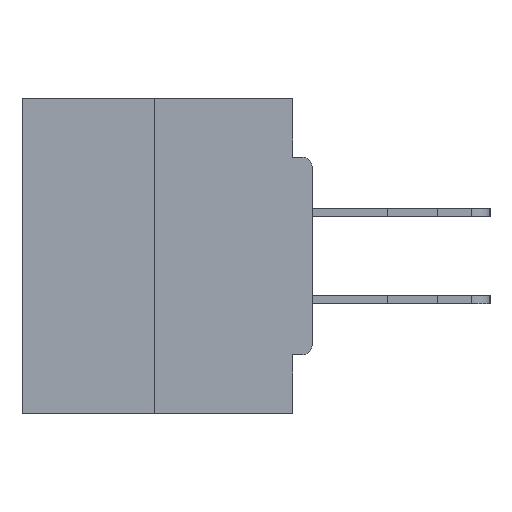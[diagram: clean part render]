
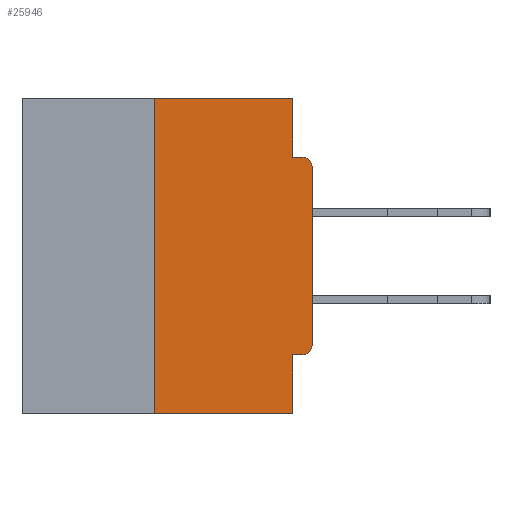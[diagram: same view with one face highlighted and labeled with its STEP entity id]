
A CAD part, left-side view. The second image highlights one B-rep face of the part: STEP entity #25946.
In plain terms, the highlighted planar face has unit normal (-1, 0, 0).
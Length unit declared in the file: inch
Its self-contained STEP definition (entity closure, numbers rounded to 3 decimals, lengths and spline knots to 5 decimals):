
#322 = VECTOR ( 'NONE', #29726, 39.37008 ) ;
#1037 = VERTEX_POINT ( 'NONE', #26358 ) ;
#1400 = VECTOR ( 'NONE', #1673, 39.37008 ) ;
#1673 = DIRECTION ( 'NONE',  ( 0., 0., -1. ) ) ;
#1866 = CARTESIAN_POINT ( 'NONE',  ( 0., 0.031, -0.5 ) ) ;
#2128 = CARTESIAN_POINT ( 'NONE',  ( 0., 0.25, -0.5 ) ) ;
#3166 = LINE ( 'NONE', #31218, #36652 ) ;
#3192 = VERTEX_POINT ( 'NONE', #12586 ) ;
#3571 = VECTOR ( 'NONE', #27977, 39.37008 ) ;
#4007 = VERTEX_POINT ( 'NONE', #32716 ) ;
#4703 = EDGE_LOOP ( 'NONE', ( #18840, #27995, #8814, #18042, #5369, #9398, #6115, #21637, #16506, #18083 ) ) ;
#5052 = VERTEX_POINT ( 'NONE', #2128 ) ;
#5257 = AXIS2_PLACEMENT_3D ( 'NONE', #32808, #23676, #10873 ) ;
#5369 = ORIENTED_EDGE ( 'NONE', *, *, #29770, .F. ) ;
#6115 = ORIENTED_EDGE ( 'NONE', *, *, #11020, .T. ) ;
#6342 = DIRECTION ( 'NONE',  ( 0., 1., 0. ) ) ;
#6436 = CARTESIAN_POINT ( 'NONE',  ( 0., 0.031, -0.0935 ) ) ;
#7241 = CIRCLE ( 'NONE', #5257, 0.015 ) ;
#7997 = VERTEX_POINT ( 'NONE', #20599 ) ;
#8484 = CIRCLE ( 'NONE', #36384, 0.015 ) ;
#8524 = DIRECTION ( 'NONE',  ( 0., 0., -1. ) ) ;
#8814 = ORIENTED_EDGE ( 'NONE', *, *, #34856, .T. ) ;
#8914 = PLANE ( 'NONE',  #25344 ) ;
#9200 = VERTEX_POINT ( 'NONE', #6436 ) ;
#9283 = EDGE_CURVE ( 'NONE', #3192, #9200, #27256, .T. ) ;
#9398 = ORIENTED_EDGE ( 'NONE', *, *, #17952, .T. ) ;
#9691 = DIRECTION ( 'NONE',  ( -1., 0., 0. ) ) ;
#10873 = DIRECTION ( 'NONE',  ( 0., 0., -1. ) ) ;
#11020 = EDGE_CURVE ( 'NONE', #1037, #33660, #17068, .T. ) ;
#12321 = CARTESIAN_POINT ( 'NONE',  ( 0., 0.46, -0.5 ) ) ;
#12525 = VERTEX_POINT ( 'NONE', #18165 ) ;
#12586 = CARTESIAN_POINT ( 'NONE',  ( 0., 0.031, 0. ) ) ;
#16506 = ORIENTED_EDGE ( 'NONE', *, *, #16971, .F. ) ;
#16971 = EDGE_CURVE ( 'NONE', #9200, #12525, #34579, .T. ) ;
#17068 = LINE ( 'NONE', #26404, #28791 ) ;
#17894 = CARTESIAN_POINT ( 'NONE',  ( 0., 0.46, 0. ) ) ;
#17921 = DIRECTION ( 'NONE',  ( 0., 0., -1. ) ) ;
#17952 = EDGE_CURVE ( 'NONE', #7997, #1037, #8484, .T. ) ;
#18042 = ORIENTED_EDGE ( 'NONE', *, *, #27162, .F. ) ;
#18083 = ORIENTED_EDGE ( 'NONE', *, *, #9283, .F. ) ;
#18100 = FACE_OUTER_BOUND ( 'NONE', #4703, .T. ) ;
#18165 = CARTESIAN_POINT ( 'NONE',  ( 0., 0.015, -0.0935 ) ) ;
#18563 = VERTEX_POINT ( 'NONE', #33606 ) ;
#18840 = ORIENTED_EDGE ( 'NONE', *, *, #23369, .F. ) ;
#19565 = DIRECTION ( 'NONE',  ( 0., -1., 0. ) ) ;
#19803 = CARTESIAN_POINT ( 'NONE',  ( 0., 0.25, 0. ) ) ;
#20599 = CARTESIAN_POINT ( 'NONE',  ( 0., 0.015, -0.4065 ) ) ;
#21637 = ORIENTED_EDGE ( 'NONE', *, *, #26732, .T. ) ;
#22120 = EDGE_CURVE ( 'NONE', #5052, #18563, #29320, .T. ) ;
#23369 = EDGE_CURVE ( 'NONE', #18563, #3192, #3166, .T. ) ;
#23676 = DIRECTION ( 'NONE',  ( -1., 0., 0. ) ) ;
#24653 = VECTOR ( 'NONE', #19565, 39.37008 ) ;
#25130 = LINE ( 'NONE', #12321, #3571 ) ;
#25156 = CARTESIAN_POINT ( 'NONE',  ( 0., 0.015, -0.3915 ) ) ;
#25344 = AXIS2_PLACEMENT_3D ( 'NONE', #17894, #27637, #8524 ) ;
#25439 = CARTESIAN_POINT ( 'NONE',  ( 0., 0., -0.4065 ) ) ;
#25453 = VECTOR ( 'NONE', #17921, 39.37008 ) ;
#25838 = CARTESIAN_POINT ( 'NONE',  ( 0., 0.031, -0.4065 ) ) ;
#25946 = ADVANCED_FACE ( 'NONE', ( #18100 ), #8914, .F. ) ;
#26358 = CARTESIAN_POINT ( 'NONE',  ( 0., 0., -0.3915 ) ) ;
#26404 = CARTESIAN_POINT ( 'NONE',  ( 0., 0., 0. ) ) ;
#26732 = EDGE_CURVE ( 'NONE', #33660, #12525, #7241, .T. ) ;
#27162 = EDGE_CURVE ( 'NONE', #29762, #4007, #29723, .T. ) ;
#27256 = LINE ( 'NONE', #30297, #25453 ) ;
#27637 = DIRECTION ( 'NONE',  ( 1., 0., 0. ) ) ;
#27977 = DIRECTION ( 'NONE',  ( 0., -1., 0. ) ) ;
#27995 = ORIENTED_EDGE ( 'NONE', *, *, #22120, .F. ) ;
#28791 = VECTOR ( 'NONE', #32682, 39.37008 ) ;
#28797 = DIRECTION ( 'NONE',  ( 0., 0., -1. ) ) ;
#29320 = LINE ( 'NONE', #19803, #322 ) ;
#29723 = LINE ( 'NONE', #1866, #1400 ) ;
#29726 = DIRECTION ( 'NONE',  ( 0., 0., 1. ) ) ;
#29762 = VERTEX_POINT ( 'NONE', #25838 ) ;
#29770 = EDGE_CURVE ( 'NONE', #7997, #29762, #38218, .T. ) ;
#30297 = CARTESIAN_POINT ( 'NONE',  ( 0., 0.031, 0. ) ) ;
#31218 = CARTESIAN_POINT ( 'NONE',  ( 0., 0.46, 0. ) ) ;
#32682 = DIRECTION ( 'NONE',  ( 0., 0., 1. ) ) ;
#32716 = CARTESIAN_POINT ( 'NONE',  ( 0., 0.031, -0.5 ) ) ;
#32808 = CARTESIAN_POINT ( 'NONE',  ( 0., 0.015, -0.1085 ) ) ;
#33606 = CARTESIAN_POINT ( 'NONE',  ( 0., 0.25, 0. ) ) ;
#33660 = VERTEX_POINT ( 'NONE', #38858 ) ;
#34579 = LINE ( 'NONE', #38232, #24653 ) ;
#34856 = EDGE_CURVE ( 'NONE', #5052, #4007, #25130, .T. ) ;
#35875 = VECTOR ( 'NONE', #6342, 39.37008 ) ;
#36384 = AXIS2_PLACEMENT_3D ( 'NONE', #25156, #9691, #28797 ) ;
#36652 = VECTOR ( 'NONE', #37510, 39.37008 ) ;
#37510 = DIRECTION ( 'NONE',  ( 0., -1., 0. ) ) ;
#38218 = LINE ( 'NONE', #25439, #35875 ) ;
#38232 = CARTESIAN_POINT ( 'NONE',  ( 0., 0., -0.0935 ) ) ;
#38858 = CARTESIAN_POINT ( 'NONE',  ( 0., 0., -0.1085 ) ) ;
